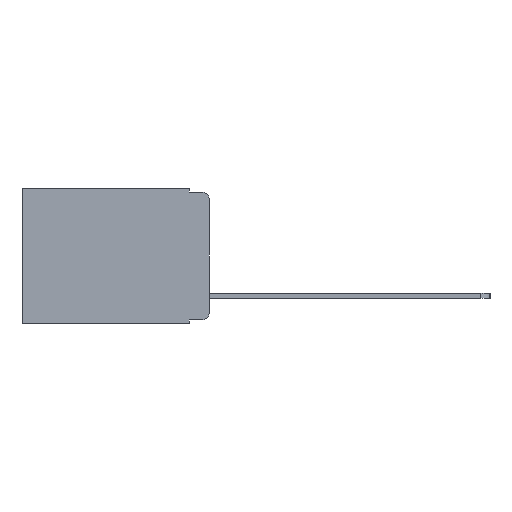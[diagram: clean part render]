
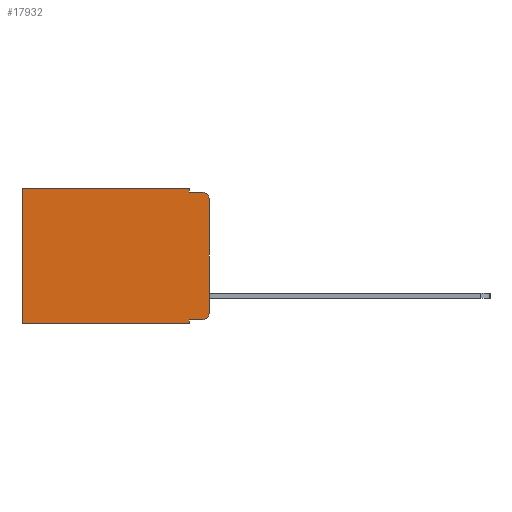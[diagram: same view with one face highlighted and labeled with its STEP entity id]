
A CAD part, left-side view. The second image highlights one B-rep face of the part: STEP entity #17932.
In plain terms, the highlighted planar face has unit normal (-1, 0, 0).
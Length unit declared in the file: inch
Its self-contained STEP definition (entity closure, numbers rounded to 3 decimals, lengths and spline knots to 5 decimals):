
#188 = ORIENTED_EDGE ( 'NONE', *, *, #10000, .F. ) ;
#845 = VERTEX_POINT ( 'NONE', #8220 ) ;
#1548 = LINE ( 'NONE', #2022, #16166 ) ;
#1635 = CARTESIAN_POINT ( 'NONE',  ( 0.298, 0.473, 0. ) ) ;
#1792 = ORIENTED_EDGE ( 'NONE', *, *, #17773, .F. ) ;
#1939 = AXIS2_PLACEMENT_3D ( 'NONE', #6749, #16030, #8116 ) ;
#2022 = CARTESIAN_POINT ( 'NONE',  ( 0.298, 0.051, 0. ) ) ;
#2059 = VECTOR ( 'NONE', #16698, 39.37008 ) ;
#2394 = EDGE_CURVE ( 'NONE', #7278, #845, #9650, .T. ) ;
#2792 = CARTESIAN_POINT ( 'NONE',  ( 0.298, 0.051, 0. ) ) ;
#2847 = CARTESIAN_POINT ( 'NONE',  ( 0.298, 0., 0. ) ) ;
#3339 = LINE ( 'NONE', #15045, #17221 ) ;
#3684 = CARTESIAN_POINT ( 'NONE',  ( 0.298, 0.051, -0.01 ) ) ;
#4318 = LINE ( 'NONE', #2792, #8458 ) ;
#4337 = VERTEX_POINT ( 'NONE', #10501 ) ;
#4803 = VERTEX_POINT ( 'NONE', #3684 ) ;
#5245 = VERTEX_POINT ( 'NONE', #1635 ) ;
#5411 = EDGE_CURVE ( 'NONE', #845, #15534, #11298, .T. ) ;
#6192 = CARTESIAN_POINT ( 'NONE',  ( 0.298, 0.051, -0.343 ) ) ;
#6339 = EDGE_CURVE ( 'NONE', #7278, #13755, #1548, .T. ) ;
#6366 = CARTESIAN_POINT ( 'NONE',  ( 0.298, 0.02, -0.313 ) ) ;
#6749 = CARTESIAN_POINT ( 'NONE',  ( 0.298, 0.02, -0.03 ) ) ;
#6939 = LINE ( 'NONE', #17240, #10145 ) ;
#7240 = EDGE_CURVE ( 'NONE', #5245, #8560, #7698, .T. ) ;
#7259 = ORIENTED_EDGE ( 'NONE', *, *, #7240, .T. ) ;
#7278 = VERTEX_POINT ( 'NONE', #14500 ) ;
#7698 = LINE ( 'NONE', #14447, #14039 ) ;
#7721 = DIRECTION ( 'NONE',  ( 0., 0., -1. ) ) ;
#7758 = DIRECTION ( 'NONE',  ( 0., 0., -1. ) ) ;
#8084 = DIRECTION ( 'NONE',  ( 0., 0., -1. ) ) ;
#8113 = ORIENTED_EDGE ( 'NONE', *, *, #10314, .T. ) ;
#8116 = DIRECTION ( 'NONE',  ( 0., 0., -1. ) ) ;
#8220 = CARTESIAN_POINT ( 'NONE',  ( 0.298, 0.02, -0.333 ) ) ;
#8423 = DIRECTION ( 'NONE',  ( 0., -1., 0. ) ) ;
#8458 = VECTOR ( 'NONE', #12512, 39.37008 ) ;
#8471 = AXIS2_PLACEMENT_3D ( 'NONE', #14755, #16002, #8084 ) ;
#8553 = DIRECTION ( 'NONE',  ( 0., 0., -1. ) ) ;
#8555 = ORIENTED_EDGE ( 'NONE', *, *, #14459, .T. ) ;
#8560 = VERTEX_POINT ( 'NONE', #13678 ) ;
#8653 = CARTESIAN_POINT ( 'NONE',  ( 0.298, 0., -0.343 ) ) ;
#8672 = LINE ( 'NONE', #8653, #11812 ) ;
#9573 = EDGE_CURVE ( 'NONE', #13755, #8560, #8672, .T. ) ;
#9650 = LINE ( 'NONE', #10014, #2059 ) ;
#10000 = EDGE_CURVE ( 'NONE', #11158, #4803, #4318, .T. ) ;
#10014 = CARTESIAN_POINT ( 'NONE',  ( 0.298, 0.051, -0.333 ) ) ;
#10145 = VECTOR ( 'NONE', #12079, 39.37008 ) ;
#10314 = EDGE_CURVE ( 'NONE', #11158, #5245, #6939, .T. ) ;
#10433 = ORIENTED_EDGE ( 'NONE', *, *, #2394, .T. ) ;
#10501 = CARTESIAN_POINT ( 'NONE',  ( 0.298, 0., -0.03 ) ) ;
#10667 = ORIENTED_EDGE ( 'NONE', *, *, #5411, .T. ) ;
#10855 = EDGE_CURVE ( 'NONE', #4803, #17307, #3339, .T. ) ;
#11031 = FACE_OUTER_BOUND ( 'NONE', #11096, .T. ) ;
#11096 = EDGE_LOOP ( 'NONE', ( #1792, #8555, #12126, #188, #8113, #7259, #14419, #16944, #10433, #10667 ) ) ;
#11158 = VERTEX_POINT ( 'NONE', #14595 ) ;
#11276 = DIRECTION ( 'NONE',  ( 0., 1., 0. ) ) ;
#11298 = CIRCLE ( 'NONE', #14438, 0.02 ) ;
#11812 = VECTOR ( 'NONE', #11276, 39.37008 ) ;
#12079 = DIRECTION ( 'NONE',  ( 0., 1., 0. ) ) ;
#12126 = ORIENTED_EDGE ( 'NONE', *, *, #10855, .F. ) ;
#12512 = DIRECTION ( 'NONE',  ( 0., 0., -1. ) ) ;
#12746 = VECTOR ( 'NONE', #8553, 39.37008 ) ;
#13454 = PLANE ( 'NONE',  #8471 ) ;
#13678 = CARTESIAN_POINT ( 'NONE',  ( 0.298, 0.473, -0.343 ) ) ;
#13755 = VERTEX_POINT ( 'NONE', #6192 ) ;
#14039 = VECTOR ( 'NONE', #15695, 39.37008 ) ;
#14419 = ORIENTED_EDGE ( 'NONE', *, *, #9573, .F. ) ;
#14438 = AXIS2_PLACEMENT_3D ( 'NONE', #6366, #15678, #7721 ) ;
#14447 = CARTESIAN_POINT ( 'NONE',  ( 0.298, 0.473, 0. ) ) ;
#14459 = EDGE_CURVE ( 'NONE', #4337, #17307, #15337, .T. ) ;
#14474 = CARTESIAN_POINT ( 'NONE',  ( 0.298, 0.02, -0.01 ) ) ;
#14500 = CARTESIAN_POINT ( 'NONE',  ( 0.298, 0.051, -0.333 ) ) ;
#14595 = CARTESIAN_POINT ( 'NONE',  ( 0.298, 0.051, 0. ) ) ;
#14755 = CARTESIAN_POINT ( 'NONE',  ( 0.298, 0., 0. ) ) ;
#15045 = CARTESIAN_POINT ( 'NONE',  ( 0.298, 0.051, -0.01 ) ) ;
#15337 = CIRCLE ( 'NONE', #1939, 0.02 ) ;
#15534 = VERTEX_POINT ( 'NONE', #16709 ) ;
#15678 = DIRECTION ( 'NONE',  ( -1., 0., 0. ) ) ;
#15695 = DIRECTION ( 'NONE',  ( 0., 0., -1. ) ) ;
#16002 = DIRECTION ( 'NONE',  ( 1., 0., 0. ) ) ;
#16030 = DIRECTION ( 'NONE',  ( -1., 0., 0. ) ) ;
#16148 = LINE ( 'NONE', #2847, #12746 ) ;
#16166 = VECTOR ( 'NONE', #7758, 39.37008 ) ;
#16698 = DIRECTION ( 'NONE',  ( 0., -1., 0. ) ) ;
#16709 = CARTESIAN_POINT ( 'NONE',  ( 0.298, 0., -0.313 ) ) ;
#16944 = ORIENTED_EDGE ( 'NONE', *, *, #6339, .F. ) ;
#17221 = VECTOR ( 'NONE', #8423, 39.37008 ) ;
#17240 = CARTESIAN_POINT ( 'NONE',  ( 0.298, 0., 0. ) ) ;
#17307 = VERTEX_POINT ( 'NONE', #14474 ) ;
#17773 = EDGE_CURVE ( 'NONE', #4337, #15534, #16148, .T. ) ;
#17932 = ADVANCED_FACE ( 'NONE', ( #11031 ), #13454, .F. ) ;
